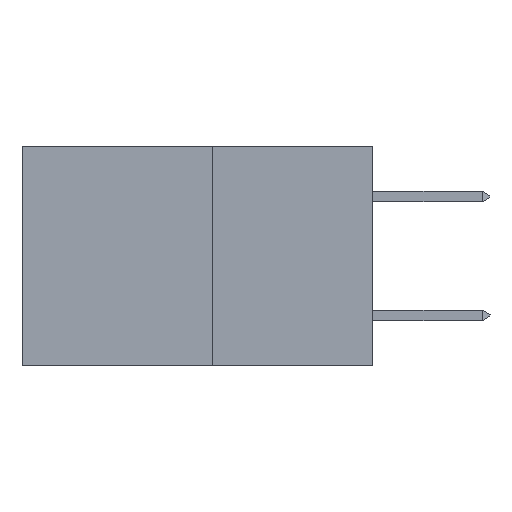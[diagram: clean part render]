
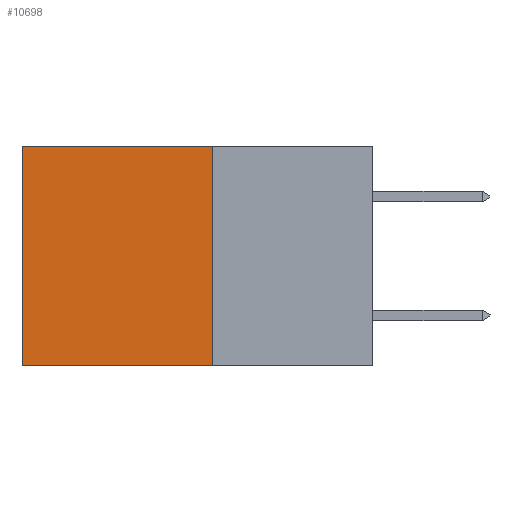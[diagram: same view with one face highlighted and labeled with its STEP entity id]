
A CAD part, left-side view. The second image highlights one B-rep face of the part: STEP entity #10698.
In plain terms, the highlighted planar face has unit normal (-1, 0, 0).
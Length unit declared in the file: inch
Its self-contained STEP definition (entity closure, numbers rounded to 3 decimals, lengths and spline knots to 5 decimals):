
#1515 = DIRECTION ( 'NONE',  ( 0., 0., -1. ) ) ;
#2473 = LINE ( 'NONE', #9808, #15970 ) ;
#3428 = DIRECTION ( 'NONE',  ( 0., 1., 0. ) ) ;
#3521 = AXIS2_PLACEMENT_3D ( 'NONE', #23896, #8861, #26353 ) ;
#3536 = CARTESIAN_POINT ( 'NONE',  ( 0.277, 0.27, 0. ) ) ;
#5619 = EDGE_CURVE ( 'NONE', #10629, #19802, #12975, .T. ) ;
#6170 = CARTESIAN_POINT ( 'NONE',  ( 0.277, 0.27, -0.37 ) ) ;
#6312 = PLANE ( 'NONE',  #3521 ) ;
#7014 = VECTOR ( 'NONE', #26211, 39.37008 ) ;
#8861 = DIRECTION ( 'NONE',  ( 1., 0., 0. ) ) ;
#9217 = CARTESIAN_POINT ( 'NONE',  ( 0.277, 0.59, -0.37 ) ) ;
#9808 = CARTESIAN_POINT ( 'NONE',  ( 0.277, 0.27, -0.37 ) ) ;
#10629 = VERTEX_POINT ( 'NONE', #3536 ) ;
#10698 = ADVANCED_FACE ( 'NONE', ( #16965 ), #6312, .F. ) ;
#12222 = LINE ( 'NONE', #21570, #24706 ) ;
#12975 = LINE ( 'NONE', #6170, #7014 ) ;
#13999 = EDGE_CURVE ( 'NONE', #10629, #24630, #28941, .T. ) ;
#15457 = ORIENTED_EDGE ( 'NONE', *, *, #13999, .T. ) ;
#15970 = VECTOR ( 'NONE', #27235, 39.37008 ) ;
#16965 = FACE_OUTER_BOUND ( 'NONE', #28107, .T. ) ;
#17628 = VERTEX_POINT ( 'NONE', #9217 ) ;
#17781 = ORIENTED_EDGE ( 'NONE', *, *, #22355, .F. ) ;
#19418 = EDGE_CURVE ( 'NONE', #24630, #17628, #12222, .T. ) ;
#19802 = VERTEX_POINT ( 'NONE', #25407 ) ;
#21092 = CARTESIAN_POINT ( 'NONE',  ( 0.277, 0.27, 0. ) ) ;
#21570 = CARTESIAN_POINT ( 'NONE',  ( 0.277, 0.59, -0.37 ) ) ;
#21623 = VECTOR ( 'NONE', #3428, 39.37008 ) ;
#22355 = EDGE_CURVE ( 'NONE', #19802, #17628, #2473, .T. ) ;
#23896 = CARTESIAN_POINT ( 'NONE',  ( 0.277, 0.27, -0.37 ) ) ;
#24580 = ORIENTED_EDGE ( 'NONE', *, *, #5619, .F. ) ;
#24630 = VERTEX_POINT ( 'NONE', #29167 ) ;
#24706 = VECTOR ( 'NONE', #1515, 39.37008 ) ;
#25407 = CARTESIAN_POINT ( 'NONE',  ( 0.277, 0.27, -0.37 ) ) ;
#26211 = DIRECTION ( 'NONE',  ( 0., 0., -1. ) ) ;
#26353 = DIRECTION ( 'NONE',  ( 0., 0., -1. ) ) ;
#27235 = DIRECTION ( 'NONE',  ( 0., 1., 0. ) ) ;
#28107 = EDGE_LOOP ( 'NONE', ( #29622, #17781, #24580, #15457 ) ) ;
#28941 = LINE ( 'NONE', #21092, #21623 ) ;
#29167 = CARTESIAN_POINT ( 'NONE',  ( 0.277, 0.59, 0. ) ) ;
#29622 = ORIENTED_EDGE ( 'NONE', *, *, #19418, .T. ) ;
